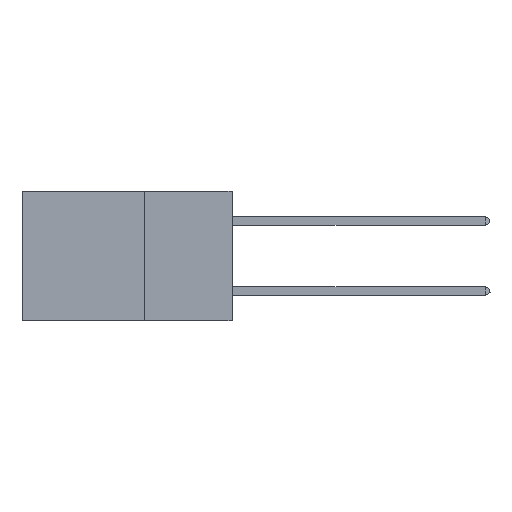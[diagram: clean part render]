
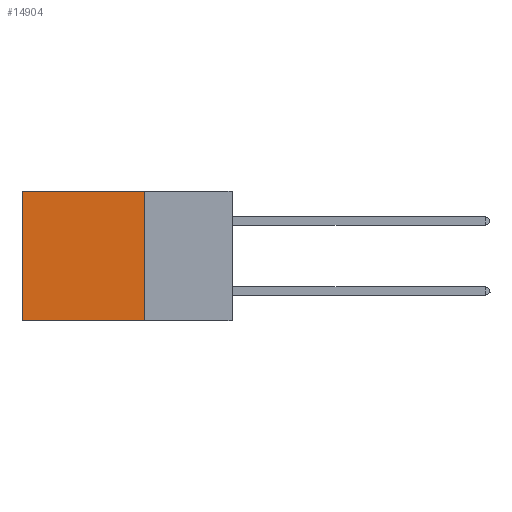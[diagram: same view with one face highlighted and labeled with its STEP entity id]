
A CAD part, left-side view. The second image highlights one B-rep face of the part: STEP entity #14904.
In plain terms, the highlighted planar face has unit normal (-1, 0, 0).
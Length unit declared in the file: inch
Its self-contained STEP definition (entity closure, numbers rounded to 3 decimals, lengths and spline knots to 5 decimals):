
#476 = PLANE ( 'NONE',  #9420 ) ;
#585 = DIRECTION ( 'NONE',  ( 0., 1., 0. ) ) ;
#1881 = DIRECTION ( 'NONE',  ( 0., 0., -1. ) ) ;
#3238 = LINE ( 'NONE', #15038, #13925 ) ;
#3262 = ORIENTED_EDGE ( 'NONE', *, *, #13635, .T. ) ;
#4342 = VECTOR ( 'NONE', #8646, 39.37008 ) ;
#4433 = EDGE_CURVE ( 'NONE', #9976, #15319, #3238, .T. ) ;
#5259 = CARTESIAN_POINT ( 'NONE',  ( 0.2875, 0.6, 0. ) ) ;
#5841 = CARTESIAN_POINT ( 'NONE',  ( 0.2875, 0.25, 0. ) ) ;
#6200 = EDGE_LOOP ( 'NONE', ( #3262, #14378, #12103, #10423 ) ) ;
#8228 = EDGE_CURVE ( 'NONE', #18116, #10091, #9565, .T. ) ;
#8459 = DIRECTION ( 'NONE',  ( 0., 0., -1. ) ) ;
#8613 = CARTESIAN_POINT ( 'NONE',  ( 0.2875, 0.25, -0.37 ) ) ;
#8646 = DIRECTION ( 'NONE',  ( 0., 0., -1. ) ) ;
#8824 = LINE ( 'NONE', #5841, #16549 ) ;
#9033 = LINE ( 'NONE', #16671, #4342 ) ;
#9227 = CARTESIAN_POINT ( 'NONE',  ( 0.2875, 0.25, -0.37 ) ) ;
#9420 = AXIS2_PLACEMENT_3D ( 'NONE', #11978, #13466, #1881 ) ;
#9565 = LINE ( 'NONE', #8613, #17993 ) ;
#9913 = CARTESIAN_POINT ( 'NONE',  ( 0.2875, 0.6, -0.37 ) ) ;
#9976 = VERTEX_POINT ( 'NONE', #12495 ) ;
#10091 = VERTEX_POINT ( 'NONE', #9913 ) ;
#10423 = ORIENTED_EDGE ( 'NONE', *, *, #4433, .T. ) ;
#11414 = FACE_OUTER_BOUND ( 'NONE', #6200, .T. ) ;
#11978 = CARTESIAN_POINT ( 'NONE',  ( 0.2875, 0.25, 0. ) ) ;
#12103 = ORIENTED_EDGE ( 'NONE', *, *, #13248, .F. ) ;
#12253 = DIRECTION ( 'NONE',  ( 0., 1., 0. ) ) ;
#12495 = CARTESIAN_POINT ( 'NONE',  ( 0.2875, 0.25, 0. ) ) ;
#13248 = EDGE_CURVE ( 'NONE', #9976, #18116, #8824, .T. ) ;
#13466 = DIRECTION ( 'NONE',  ( 1., 0., 0. ) ) ;
#13635 = EDGE_CURVE ( 'NONE', #15319, #10091, #9033, .T. ) ;
#13925 = VECTOR ( 'NONE', #12253, 39.37008 ) ;
#14378 = ORIENTED_EDGE ( 'NONE', *, *, #8228, .F. ) ;
#14904 = ADVANCED_FACE ( 'NONE', ( #11414 ), #476, .F. ) ;
#15038 = CARTESIAN_POINT ( 'NONE',  ( 0.2875, 0.25, 0. ) ) ;
#15319 = VERTEX_POINT ( 'NONE', #5259 ) ;
#16549 = VECTOR ( 'NONE', #8459, 39.37008 ) ;
#16671 = CARTESIAN_POINT ( 'NONE',  ( 0.2875, 0.6, 0. ) ) ;
#17993 = VECTOR ( 'NONE', #585, 39.37008 ) ;
#18116 = VERTEX_POINT ( 'NONE', #9227 ) ;
